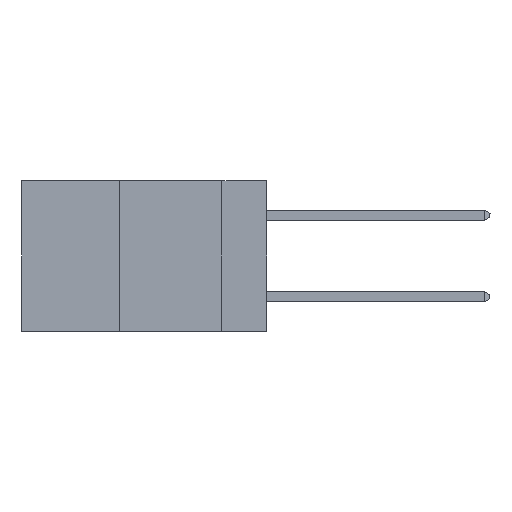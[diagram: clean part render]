
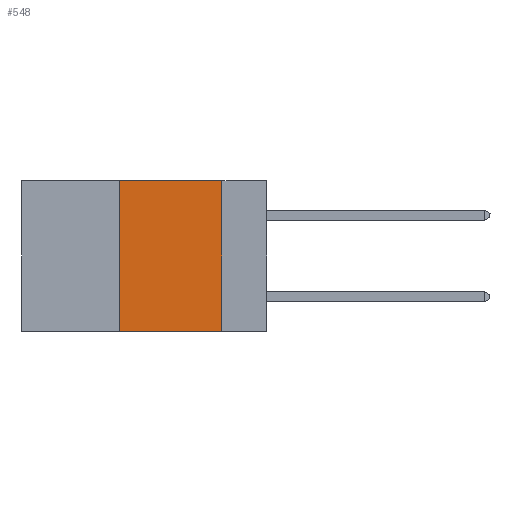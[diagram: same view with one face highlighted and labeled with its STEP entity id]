
A CAD part, left-side view. The second image highlights one B-rep face of the part: STEP entity #548.
In plain terms, the highlighted planar face has unit normal (-1, 0, 0).
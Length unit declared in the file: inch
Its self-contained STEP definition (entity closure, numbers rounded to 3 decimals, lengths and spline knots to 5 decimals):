
#548 = ADVANCED_FACE ( 'NONE', ( #11336 ), #13860, .F. ) ;
#681 = VECTOR ( 'NONE', #6368, 39.37008 ) ;
#927 = LINE ( 'NONE', #6471, #4452 ) ;
#1314 = LINE ( 'NONE', #9489, #12192 ) ;
#2129 = ORIENTED_EDGE ( 'NONE', *, *, #6136, .T. ) ;
#2301 = EDGE_CURVE ( 'NONE', #7233, #10531, #9195, .T. ) ;
#2930 = VERTEX_POINT ( 'NONE', #15028 ) ;
#3158 = CARTESIAN_POINT ( 'NONE',  ( 0., 0.36, -0.37 ) ) ;
#4082 = EDGE_LOOP ( 'NONE', ( #8733, #11786, #4149, #2129 ) ) ;
#4149 = ORIENTED_EDGE ( 'NONE', *, *, #4508, .F. ) ;
#4362 = DIRECTION ( 'NONE',  ( 1., 0., 0. ) ) ;
#4452 = VECTOR ( 'NONE', #13075, 39.37008 ) ;
#4508 = EDGE_CURVE ( 'NONE', #11156, #7233, #1314, .T. ) ;
#5535 = CARTESIAN_POINT ( 'NONE',  ( 0., 0.6, 0. ) ) ;
#6136 = EDGE_CURVE ( 'NONE', #11156, #2930, #12074, .T. ) ;
#6368 = DIRECTION ( 'NONE',  ( 0., -1., 0. ) ) ;
#6471 = CARTESIAN_POINT ( 'NONE',  ( 0., 0.11, 0. ) ) ;
#7233 = VERTEX_POINT ( 'NONE', #11987 ) ;
#7351 = EDGE_CURVE ( 'NONE', #10531, #2930, #927, .T. ) ;
#7739 = CARTESIAN_POINT ( 'NONE',  ( 0., 0.6, 0. ) ) ;
#8106 = DIRECTION ( 'NONE',  ( 0., -1., 0. ) ) ;
#8202 = VECTOR ( 'NONE', #8106, 39.37008 ) ;
#8283 = CARTESIAN_POINT ( 'NONE',  ( 0., 0.11, 0. ) ) ;
#8733 = ORIENTED_EDGE ( 'NONE', *, *, #7351, .F. ) ;
#9195 = LINE ( 'NONE', #7739, #681 ) ;
#9489 = CARTESIAN_POINT ( 'NONE',  ( 0., 0.36, 0. ) ) ;
#10531 = VERTEX_POINT ( 'NONE', #8283 ) ;
#11156 = VERTEX_POINT ( 'NONE', #3158 ) ;
#11336 = FACE_OUTER_BOUND ( 'NONE', #4082, .T. ) ;
#11786 = ORIENTED_EDGE ( 'NONE', *, *, #2301, .F. ) ;
#11987 = CARTESIAN_POINT ( 'NONE',  ( 0., 0.36, 0. ) ) ;
#12074 = LINE ( 'NONE', #14801, #8202 ) ;
#12192 = VECTOR ( 'NONE', #17918, 39.37008 ) ;
#13075 = DIRECTION ( 'NONE',  ( 0., 0., -1. ) ) ;
#13860 = PLANE ( 'NONE',  #15173 ) ;
#14801 = CARTESIAN_POINT ( 'NONE',  ( 0., 0.6, -0.37 ) ) ;
#15028 = CARTESIAN_POINT ( 'NONE',  ( 0., 0.11, -0.37 ) ) ;
#15173 = AXIS2_PLACEMENT_3D ( 'NONE', #5535, #4362, #17880 ) ;
#17880 = DIRECTION ( 'NONE',  ( 0., 0., -1. ) ) ;
#17918 = DIRECTION ( 'NONE',  ( 0., 0., 1. ) ) ;
